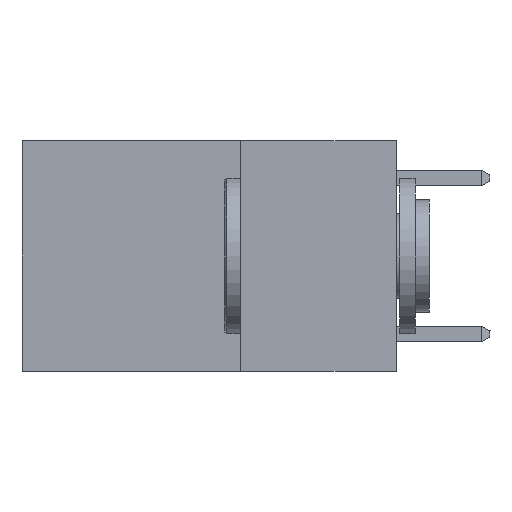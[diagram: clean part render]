
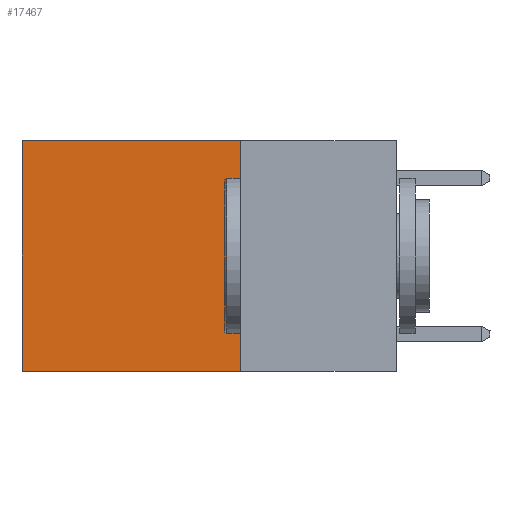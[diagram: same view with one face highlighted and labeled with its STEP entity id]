
A CAD part, left-side view. The second image highlights one B-rep face of the part: STEP entity #17467.
In plain terms, the highlighted planar face has unit normal (-1, 0, 0).
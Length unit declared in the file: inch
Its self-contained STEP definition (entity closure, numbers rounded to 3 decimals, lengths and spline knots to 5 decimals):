
#733 = ORIENTED_EDGE ( 'NONE', *, *, #16097, .F. ) ;
#984 = EDGE_LOOP ( 'NONE', ( #3084, #733, #14719, #1837 ) ) ;
#1231 = CARTESIAN_POINT ( 'NONE',  ( 0.2625, 0.25, 0. ) ) ;
#1451 = VECTOR ( 'NONE', #14197, 39.37008 ) ;
#1837 = ORIENTED_EDGE ( 'NONE', *, *, #3956, .T. ) ;
#2150 = DIRECTION ( 'NONE',  ( 0., 0., -1. ) ) ;
#3084 = ORIENTED_EDGE ( 'NONE', *, *, #18305, .T. ) ;
#3956 = EDGE_CURVE ( 'NONE', #8676, #5283, #19045, .T. ) ;
#4817 = VECTOR ( 'NONE', #16758, 39.37008 ) ;
#5283 = VERTEX_POINT ( 'NONE', #19789 ) ;
#6463 = CARTESIAN_POINT ( 'NONE',  ( 0.2625, 0.6, -0.37 ) ) ;
#6855 = CARTESIAN_POINT ( 'NONE',  ( 0.2625, 0.25, -0.37 ) ) ;
#7012 = PLANE ( 'NONE',  #14894 ) ;
#8471 = VERTEX_POINT ( 'NONE', #6855 ) ;
#8676 = VERTEX_POINT ( 'NONE', #1231 ) ;
#8831 = LINE ( 'NONE', #20156, #1451 ) ;
#9307 = EDGE_CURVE ( 'NONE', #8676, #8471, #8831, .T. ) ;
#9542 = LINE ( 'NONE', #15715, #10558 ) ;
#10011 = DIRECTION ( 'NONE',  ( 1., 0., 0. ) ) ;
#10558 = VECTOR ( 'NONE', #17198, 39.37008 ) ;
#12165 = LINE ( 'NONE', #16152, #16061 ) ;
#14197 = DIRECTION ( 'NONE',  ( 0., 0., -1. ) ) ;
#14509 = DIRECTION ( 'NONE',  ( 0., 1., 0. ) ) ;
#14719 = ORIENTED_EDGE ( 'NONE', *, *, #9307, .F. ) ;
#14894 = AXIS2_PLACEMENT_3D ( 'NONE', #19375, #10011, #2150 ) ;
#15124 = CARTESIAN_POINT ( 'NONE',  ( 0.2625, 0.25, 0. ) ) ;
#15715 = CARTESIAN_POINT ( 'NONE',  ( 0.2625, 0.6, 0. ) ) ;
#16061 = VECTOR ( 'NONE', #14509, 39.37008 ) ;
#16097 = EDGE_CURVE ( 'NONE', #8471, #19598, #12165, .T. ) ;
#16152 = CARTESIAN_POINT ( 'NONE',  ( 0.2625, 0.25, -0.37 ) ) ;
#16758 = DIRECTION ( 'NONE',  ( 0., 1., 0. ) ) ;
#17198 = DIRECTION ( 'NONE',  ( 0., 0., -1. ) ) ;
#17467 = ADVANCED_FACE ( 'NONE', ( #17898 ), #7012, .F. ) ;
#17898 = FACE_OUTER_BOUND ( 'NONE', #984, .T. ) ;
#18305 = EDGE_CURVE ( 'NONE', #5283, #19598, #9542, .T. ) ;
#19045 = LINE ( 'NONE', #15124, #4817 ) ;
#19375 = CARTESIAN_POINT ( 'NONE',  ( 0.2625, 0.25, 0. ) ) ;
#19598 = VERTEX_POINT ( 'NONE', #6463 ) ;
#19789 = CARTESIAN_POINT ( 'NONE',  ( 0.2625, 0.6, 0. ) ) ;
#20156 = CARTESIAN_POINT ( 'NONE',  ( 0.2625, 0.25, 0. ) ) ;
